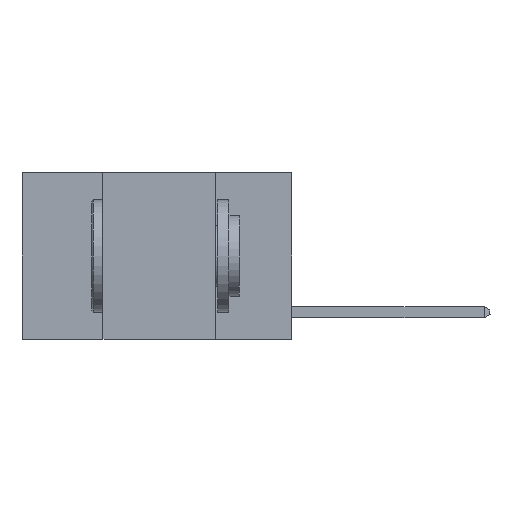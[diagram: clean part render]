
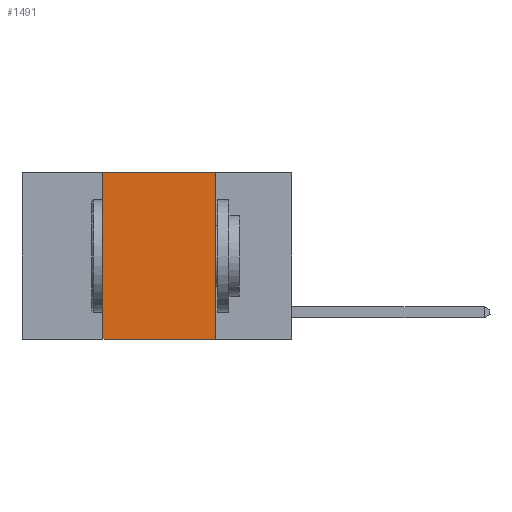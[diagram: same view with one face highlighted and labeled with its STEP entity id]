
A CAD part, left-side view. The second image highlights one B-rep face of the part: STEP entity #1491.
In plain terms, the highlighted planar face has unit normal (-1, 0, 0).
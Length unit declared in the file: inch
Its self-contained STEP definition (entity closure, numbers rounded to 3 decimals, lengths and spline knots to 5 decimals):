
#23 = VERTEX_POINT ( 'NONE', #167 ) ;
#167 = CARTESIAN_POINT ( 'NONE',  ( 0., 0.42, -0.37 ) ) ;
#1017 = VERTEX_POINT ( 'NONE', #5583 ) ;
#1344 = VECTOR ( 'NONE', #4984, 39.37008 ) ;
#1372 = VERTEX_POINT ( 'NONE', #9018 ) ;
#1491 = ADVANCED_FACE ( 'NONE', ( #3413 ), #8458, .F. ) ;
#1668 = VECTOR ( 'NONE', #6678, 39.37008 ) ;
#1923 = EDGE_CURVE ( 'NONE', #23, #1017, #8579, .T. ) ;
#1924 = EDGE_CURVE ( 'NONE', #23, #2172, #8622, .T. ) ;
#1948 = LINE ( 'NONE', #6233, #7957 ) ;
#2121 = ORIENTED_EDGE ( 'NONE', *, *, #1924, .T. ) ;
#2154 = CARTESIAN_POINT ( 'NONE',  ( 0., 0.6, 0. ) ) ;
#2172 = VERTEX_POINT ( 'NONE', #2671 ) ;
#2471 = EDGE_LOOP ( 'NONE', ( #3226, #8670, #5399, #2121 ) ) ;
#2671 = CARTESIAN_POINT ( 'NONE',  ( 0., 0.17, -0.37 ) ) ;
#2791 = DIRECTION ( 'NONE',  ( 0., 0., 1. ) ) ;
#2970 = CARTESIAN_POINT ( 'NONE',  ( 0., 0.42, 0. ) ) ;
#3226 = ORIENTED_EDGE ( 'NONE', *, *, #3962, .F. ) ;
#3413 = FACE_OUTER_BOUND ( 'NONE', #2471, .T. ) ;
#3473 = DIRECTION ( 'NONE',  ( 1., 0., 0. ) ) ;
#3557 = CARTESIAN_POINT ( 'NONE',  ( 0., 0.6, 0. ) ) ;
#3962 = EDGE_CURVE ( 'NONE', #1372, #2172, #1948, .T. ) ;
#4272 = CARTESIAN_POINT ( 'NONE',  ( 0., 0.6, -0.37 ) ) ;
#4314 = AXIS2_PLACEMENT_3D ( 'NONE', #3557, #3473, #7122 ) ;
#4984 = DIRECTION ( 'NONE',  ( 0., -1., 0. ) ) ;
#5399 = ORIENTED_EDGE ( 'NONE', *, *, #1923, .F. ) ;
#5583 = CARTESIAN_POINT ( 'NONE',  ( 0., 0.42, 0. ) ) ;
#5694 = VECTOR ( 'NONE', #2791, 39.37008 ) ;
#6233 = CARTESIAN_POINT ( 'NONE',  ( 0., 0.17, 0. ) ) ;
#6311 = EDGE_CURVE ( 'NONE', #1017, #1372, #6583, .T. ) ;
#6583 = LINE ( 'NONE', #2154, #1668 ) ;
#6678 = DIRECTION ( 'NONE',  ( 0., -1., 0. ) ) ;
#7122 = DIRECTION ( 'NONE',  ( 0., 0., -1. ) ) ;
#7957 = VECTOR ( 'NONE', #9113, 39.37008 ) ;
#8458 = PLANE ( 'NONE',  #4314 ) ;
#8579 = LINE ( 'NONE', #2970, #5694 ) ;
#8622 = LINE ( 'NONE', #4272, #1344 ) ;
#8670 = ORIENTED_EDGE ( 'NONE', *, *, #6311, .F. ) ;
#9018 = CARTESIAN_POINT ( 'NONE',  ( 0., 0.17, 0. ) ) ;
#9113 = DIRECTION ( 'NONE',  ( 0., 0., -1. ) ) ;
